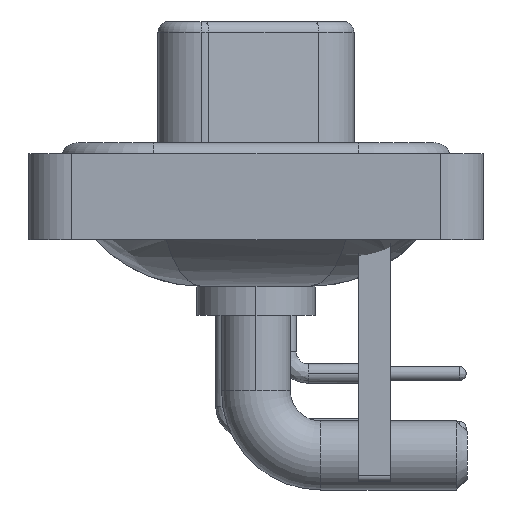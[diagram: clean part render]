
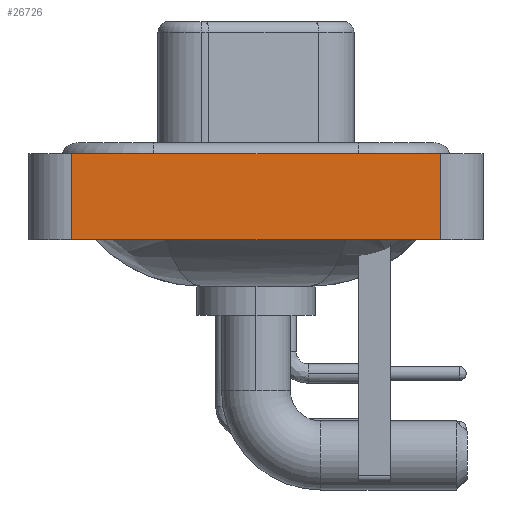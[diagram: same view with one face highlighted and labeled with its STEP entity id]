
A CAD part, left-side view. The second image highlights one B-rep face of the part: STEP entity #26726.
In plain terms, the highlighted planar face has unit normal (-1, 0, 0).
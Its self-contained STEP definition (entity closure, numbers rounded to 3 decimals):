
#837 = CARTESIAN_POINT ( 'NONE',  ( -7.35, -8.55, -3.6 ) ) ;
#2317 = ORIENTED_EDGE ( 'NONE', *, *, #21733, .F. ) ;
#2757 = CARTESIAN_POINT ( 'NONE',  ( -7.35, -8.55, -3.6 ) ) ;
#4188 = CARTESIAN_POINT ( 'NONE',  ( -7.35, -8.55, 0.4 ) ) ;
#4280 = EDGE_CURVE ( 'NONE', #5913, #21016, #6397, .T. ) ;
#4480 = CARTESIAN_POINT ( 'NONE',  ( -7.35, -8.55, 0.4 ) ) ;
#4557 = VECTOR ( 'NONE', #6270, 1000. ) ;
#4692 = VECTOR ( 'NONE', #26460, 1000. ) ;
#5913 = VERTEX_POINT ( 'NONE', #26768 ) ;
#6270 = DIRECTION ( 'NONE',  ( 0., 0., 1. ) ) ;
#6397 = LINE ( 'NONE', #17719, #7984 ) ;
#7341 = LINE ( 'NONE', #25215, #18044 ) ;
#7984 = VECTOR ( 'NONE', #15354, 1000. ) ;
#8983 = FACE_OUTER_BOUND ( 'NONE', #16869, .T. ) ;
#9272 = DIRECTION ( 'NONE',  ( 0., 0., 1. ) ) ;
#10815 = LINE ( 'NONE', #19817, #4557 ) ;
#11470 = EDGE_CURVE ( 'NONE', #21016, #19313, #7341, .T. ) ;
#11895 = ORIENTED_EDGE ( 'NONE', *, *, #11470, .T. ) ;
#15354 = DIRECTION ( 'NONE',  ( 0., -1., 0. ) ) ;
#15878 = DIRECTION ( 'NONE',  ( 0., 0., 1. ) ) ;
#16869 = EDGE_LOOP ( 'NONE', ( #11895, #27791, #2317, #18834 ) ) ;
#17719 = CARTESIAN_POINT ( 'NONE',  ( -7.35, -8.55, -3.6 ) ) ;
#18044 = VECTOR ( 'NONE', #9272, 1000. ) ;
#18834 = ORIENTED_EDGE ( 'NONE', *, *, #4280, .T. ) ;
#19299 = VERTEX_POINT ( 'NONE', #22177 ) ;
#19313 = VERTEX_POINT ( 'NONE', #4188 ) ;
#19817 = CARTESIAN_POINT ( 'NONE',  ( -7.35, 8.55, -3.6 ) ) ;
#20362 = AXIS2_PLACEMENT_3D ( 'NONE', #2757, #26978, #15878 ) ;
#21016 = VERTEX_POINT ( 'NONE', #837 ) ;
#21733 = EDGE_CURVE ( 'NONE', #5913, #19299, #10815, .T. ) ;
#22177 = CARTESIAN_POINT ( 'NONE',  ( -7.35, 8.55, 0.4 ) ) ;
#22706 = PLANE ( 'NONE',  #20362 ) ;
#24590 = EDGE_CURVE ( 'NONE', #19299, #19313, #26753, .T. ) ;
#25215 = CARTESIAN_POINT ( 'NONE',  ( -7.35, -8.55, -3.6 ) ) ;
#26460 = DIRECTION ( 'NONE',  ( 0., -1., 0. ) ) ;
#26726 = ADVANCED_FACE ( 'NONE', ( #8983 ), #22706, .T. ) ;
#26753 = LINE ( 'NONE', #4480, #4692 ) ;
#26768 = CARTESIAN_POINT ( 'NONE',  ( -7.35, 8.55, -3.6 ) ) ;
#26978 = DIRECTION ( 'NONE',  ( -1., 0., 0. ) ) ;
#27791 = ORIENTED_EDGE ( 'NONE', *, *, #24590, .F. ) ;
